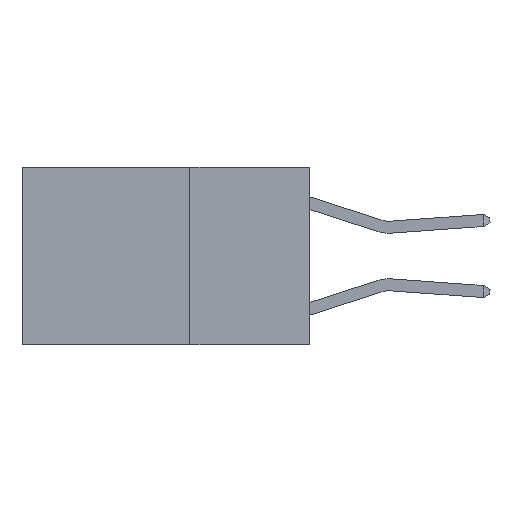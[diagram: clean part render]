
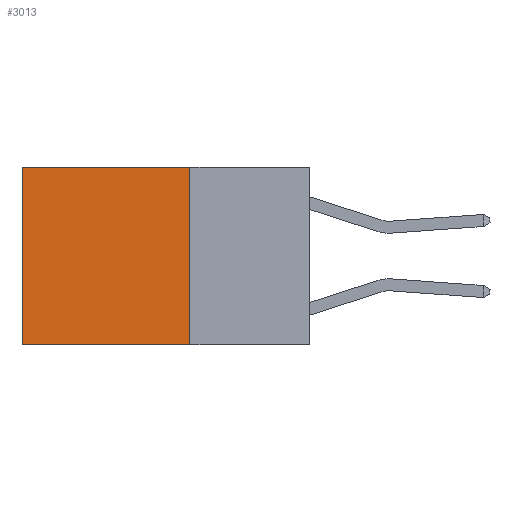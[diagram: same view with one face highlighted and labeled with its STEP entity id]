
A CAD part, left-side view. The second image highlights one B-rep face of the part: STEP entity #3013.
In plain terms, the highlighted planar face has unit normal (-1, 0, 0).
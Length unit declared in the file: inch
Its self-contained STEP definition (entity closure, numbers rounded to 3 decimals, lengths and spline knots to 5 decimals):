
#60 = EDGE_LOOP ( 'NONE', ( #2069, #6761, #4229, #4894 ) ) ;
#263 = EDGE_CURVE ( 'NONE', #7733, #3607, #6530, .T. ) ;
#312 = CARTESIAN_POINT ( 'NONE',  ( 0.2625, 0.25, 0. ) ) ;
#569 = EDGE_CURVE ( 'NONE', #5110, #5800, #7327, .T. ) ;
#990 = DIRECTION ( 'NONE',  ( 1., 0., 0. ) ) ;
#992 = PLANE ( 'NONE',  #3902 ) ;
#1076 = DIRECTION ( 'NONE',  ( 0., 0., -1. ) ) ;
#1360 = CARTESIAN_POINT ( 'NONE',  ( 0.2625, 0.25, 0. ) ) ;
#1559 = DIRECTION ( 'NONE',  ( 0., 1., 0. ) ) ;
#1849 = LINE ( 'NONE', #312, #7007 ) ;
#2069 = ORIENTED_EDGE ( 'NONE', *, *, #263, .T. ) ;
#2110 = VECTOR ( 'NONE', #1559, 39.37008 ) ;
#2551 = VECTOR ( 'NONE', #3778, 39.37008 ) ;
#2807 = CARTESIAN_POINT ( 'NONE',  ( 0.2625, 0.6, -0.37 ) ) ;
#3013 = ADVANCED_FACE ( 'NONE', ( #5443 ), #992, .F. ) ;
#3607 = VERTEX_POINT ( 'NONE', #2807 ) ;
#3778 = DIRECTION ( 'NONE',  ( 0., 0., -1. ) ) ;
#3815 = CARTESIAN_POINT ( 'NONE',  ( 0.2625, 0.6, 0. ) ) ;
#3892 = CARTESIAN_POINT ( 'NONE',  ( 0.2625, 0.25, 0. ) ) ;
#3902 = AXIS2_PLACEMENT_3D ( 'NONE', #1360, #990, #1076 ) ;
#3919 = LINE ( 'NONE', #8179, #2110 ) ;
#4229 = ORIENTED_EDGE ( 'NONE', *, *, #569, .F. ) ;
#4450 = DIRECTION ( 'NONE',  ( 0., 1., 0. ) ) ;
#4757 = CARTESIAN_POINT ( 'NONE',  ( 0.2625, 0.25, -0.37 ) ) ;
#4894 = ORIENTED_EDGE ( 'NONE', *, *, #6589, .T. ) ;
#4955 = EDGE_CURVE ( 'NONE', #5800, #3607, #3919, .T. ) ;
#5110 = VERTEX_POINT ( 'NONE', #5111 ) ;
#5111 = CARTESIAN_POINT ( 'NONE',  ( 0.2625, 0.25, 0. ) ) ;
#5443 = FACE_OUTER_BOUND ( 'NONE', #60, .T. ) ;
#5800 = VERTEX_POINT ( 'NONE', #4757 ) ;
#6530 = LINE ( 'NONE', #3815, #2551 ) ;
#6589 = EDGE_CURVE ( 'NONE', #5110, #7733, #1849, .T. ) ;
#6761 = ORIENTED_EDGE ( 'NONE', *, *, #4955, .F. ) ;
#7007 = VECTOR ( 'NONE', #4450, 39.37008 ) ;
#7138 = VECTOR ( 'NONE', #7478, 39.37008 ) ;
#7327 = LINE ( 'NONE', #3892, #7138 ) ;
#7478 = DIRECTION ( 'NONE',  ( 0., 0., -1. ) ) ;
#7733 = VERTEX_POINT ( 'NONE', #8192 ) ;
#8179 = CARTESIAN_POINT ( 'NONE',  ( 0.2625, 0.25, -0.37 ) ) ;
#8192 = CARTESIAN_POINT ( 'NONE',  ( 0.2625, 0.6, 0. ) ) ;
